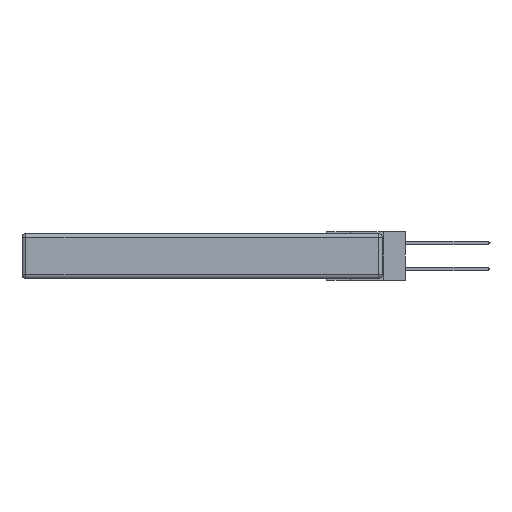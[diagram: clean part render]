
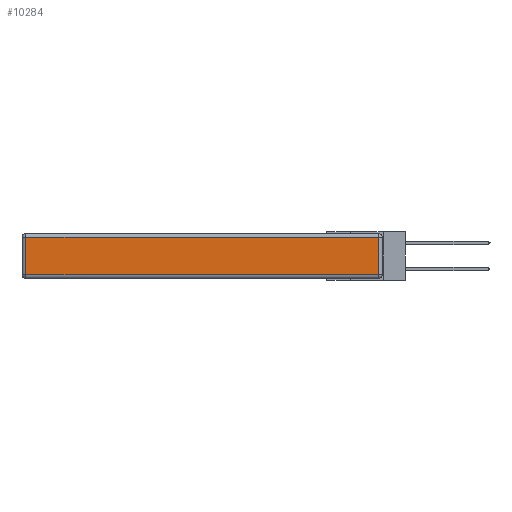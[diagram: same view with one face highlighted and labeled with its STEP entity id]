
A CAD part, left-side view. The second image highlights one B-rep face of the part: STEP entity #10284.
In plain terms, the highlighted planar face has unit normal (-1, 0, 0).
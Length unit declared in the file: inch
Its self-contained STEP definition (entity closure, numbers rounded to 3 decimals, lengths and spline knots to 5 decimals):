
#353 = VECTOR ( 'NONE', #19601, 39.37008 ) ;
#495 = EDGE_CURVE ( 'NONE', #3179, #12957, #14430, .T. ) ;
#631 = CARTESIAN_POINT ( 'NONE',  ( 0., 2.72, -0.03 ) ) ;
#2831 = CARTESIAN_POINT ( 'NONE',  ( 0., 0., -0.343 ) ) ;
#3179 = VERTEX_POINT ( 'NONE', #17664 ) ;
#3382 = VERTEX_POINT ( 'NONE', #631 ) ;
#3812 = ORIENTED_EDGE ( 'NONE', *, *, #13494, .T. ) ;
#4297 = PLANE ( 'NONE',  #16740 ) ;
#4354 = CARTESIAN_POINT ( 'NONE',  ( 0., 2.72, -0.343 ) ) ;
#4581 = VECTOR ( 'NONE', #18494, 39.37008 ) ;
#5039 = VERTEX_POINT ( 'NONE', #16459 ) ;
#5792 = CARTESIAN_POINT ( 'NONE',  ( 0., 0.03, -0.343 ) ) ;
#6249 = EDGE_CURVE ( 'NONE', #12957, #5039, #16520, .T. ) ;
#6843 = EDGE_LOOP ( 'NONE', ( #16148, #7782, #3812, #16755 ) ) ;
#7055 = CARTESIAN_POINT ( 'NONE',  ( 0., 0.03, -0.313 ) ) ;
#7374 = VECTOR ( 'NONE', #16413, 39.37008 ) ;
#7782 = ORIENTED_EDGE ( 'NONE', *, *, #6249, .T. ) ;
#8782 = DIRECTION ( 'NONE',  ( 0., 0., 1. ) ) ;
#10284 = ADVANCED_FACE ( 'NONE', ( #18852 ), #4297, .T. ) ;
#11916 = LINE ( 'NONE', #18124, #353 ) ;
#11953 = LINE ( 'NONE', #4354, #19436 ) ;
#12240 = CARTESIAN_POINT ( 'NONE',  ( 0., 0., -0.313 ) ) ;
#12957 = VERTEX_POINT ( 'NONE', #7055 ) ;
#13494 = EDGE_CURVE ( 'NONE', #5039, #3382, #11916, .T. ) ;
#14430 = LINE ( 'NONE', #12240, #4581 ) ;
#16148 = ORIENTED_EDGE ( 'NONE', *, *, #495, .T. ) ;
#16413 = DIRECTION ( 'NONE',  ( 0., 0., 1. ) ) ;
#16459 = CARTESIAN_POINT ( 'NONE',  ( 0., 0.03, -0.03 ) ) ;
#16520 = LINE ( 'NONE', #5792, #7374 ) ;
#16740 = AXIS2_PLACEMENT_3D ( 'NONE', #2831, #18030, #8782 ) ;
#16755 = ORIENTED_EDGE ( 'NONE', *, *, #18265, .T. ) ;
#17664 = CARTESIAN_POINT ( 'NONE',  ( 0., 2.72, -0.313 ) ) ;
#18030 = DIRECTION ( 'NONE',  ( -1., 0., 0. ) ) ;
#18124 = CARTESIAN_POINT ( 'NONE',  ( 0., 2.75, -0.03 ) ) ;
#18211 = DIRECTION ( 'NONE',  ( 0., 0., -1. ) ) ;
#18265 = EDGE_CURVE ( 'NONE', #3382, #3179, #11953, .T. ) ;
#18494 = DIRECTION ( 'NONE',  ( 0., -1., 0. ) ) ;
#18852 = FACE_OUTER_BOUND ( 'NONE', #6843, .T. ) ;
#19436 = VECTOR ( 'NONE', #18211, 39.37008 ) ;
#19601 = DIRECTION ( 'NONE',  ( 0., 1., 0. ) ) ;
